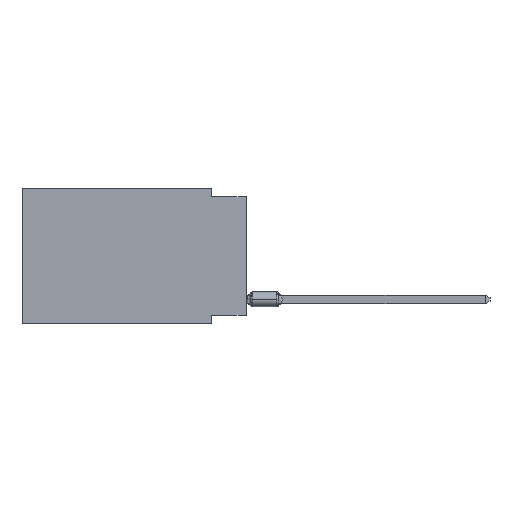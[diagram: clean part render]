
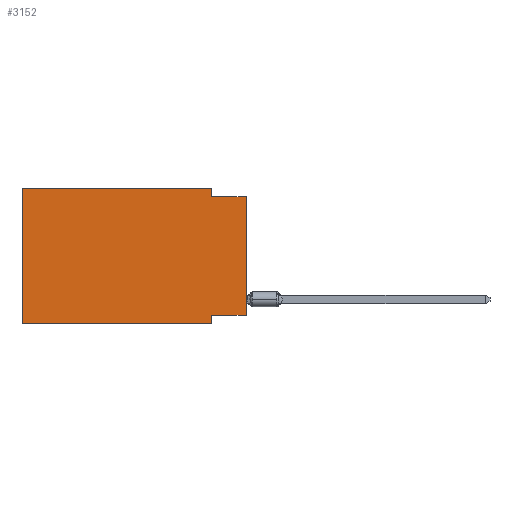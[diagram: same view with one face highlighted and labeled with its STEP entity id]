
A CAD part, left-side view. The second image highlights one B-rep face of the part: STEP entity #3152.
In plain terms, the highlighted planar face has unit normal (-1, 0, 0).
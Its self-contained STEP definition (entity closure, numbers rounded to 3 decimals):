
#295 = VERTEX_POINT ( 'NONE', #4815 ) ;
#475 = CARTESIAN_POINT ( 'NONE',  ( 0., 0., 0. ) ) ;
#758 = DIRECTION ( 'NONE',  ( 0., -1., 0. ) ) ;
#931 = VECTOR ( 'NONE', #13172, 1000. ) ;
#940 = CARTESIAN_POINT ( 'NONE',  ( 0., 16.383, 0. ) ) ;
#1069 = VECTOR ( 'NONE', #4047, 1000. ) ;
#1513 = LINE ( 'NONE', #475, #11340 ) ;
#2204 = VERTEX_POINT ( 'NONE', #8667 ) ;
#2489 = DIRECTION ( 'NONE',  ( 0., 0., -1. ) ) ;
#2542 = VECTOR ( 'NONE', #8967, 1000. ) ;
#3152 = ADVANCED_FACE ( 'NONE', ( #3897 ), #14091, .F. ) ;
#3255 = EDGE_CURVE ( 'NONE', #7846, #295, #1513, .T. ) ;
#3309 = CARTESIAN_POINT ( 'NONE',  ( 0., 0., -0.635 ) ) ;
#3440 = CARTESIAN_POINT ( 'NONE',  ( 0., 16.383, 0. ) ) ;
#3498 = CARTESIAN_POINT ( 'NONE',  ( 0., 16.383, 0. ) ) ;
#3897 = FACE_OUTER_BOUND ( 'NONE', #4303, .T. ) ;
#4021 = EDGE_CURVE ( 'NONE', #14570, #295, #4859, .T. ) ;
#4047 = DIRECTION ( 'NONE',  ( 0., 0., -1. ) ) ;
#4248 = VECTOR ( 'NONE', #12538, 1000. ) ;
#4303 = EDGE_LOOP ( 'NONE', ( #13614, #16220, #7814, #13101, #13898, #14642, #16338, #11580 ) ) ;
#4553 = DIRECTION ( 'NONE',  ( 0., 0., 1. ) ) ;
#4555 = VERTEX_POINT ( 'NONE', #12777 ) ;
#4815 = CARTESIAN_POINT ( 'NONE',  ( 0., 0., -0.635 ) ) ;
#4859 = LINE ( 'NONE', #3309, #4248 ) ;
#4900 = LINE ( 'NONE', #3440, #6877 ) ;
#6648 = DIRECTION ( 'NONE',  ( 0., 0., 1. ) ) ;
#6824 = EDGE_CURVE ( 'NONE', #14554, #16844, #4900, .T. ) ;
#6877 = VECTOR ( 'NONE', #4553, 1000. ) ;
#6938 = CARTESIAN_POINT ( 'NONE',  ( 0., 0., -9.271 ) ) ;
#7018 = LINE ( 'NONE', #9733, #13177 ) ;
#7523 = LINE ( 'NONE', #3498, #2542 ) ;
#7814 = ORIENTED_EDGE ( 'NONE', *, *, #16380, .F. ) ;
#7846 = VERTEX_POINT ( 'NONE', #11588 ) ;
#8667 = CARTESIAN_POINT ( 'NONE',  ( 0., 2.54, 0. ) ) ;
#8840 = VECTOR ( 'NONE', #2489, 1000. ) ;
#8967 = DIRECTION ( 'NONE',  ( 0., -1., 0. ) ) ;
#9119 = CARTESIAN_POINT ( 'NONE',  ( 0., 16.383, 0. ) ) ;
#9468 = EDGE_CURVE ( 'NONE', #14554, #4555, #7018, .T. ) ;
#9588 = EDGE_CURVE ( 'NONE', #16844, #2204, #7523, .T. ) ;
#9733 = CARTESIAN_POINT ( 'NONE',  ( 0., 16.383, -9.906 ) ) ;
#9786 = CARTESIAN_POINT ( 'NONE',  ( 0., 16.383, -9.906 ) ) ;
#9879 = VERTEX_POINT ( 'NONE', #10924 ) ;
#10101 = LINE ( 'NONE', #12832, #8840 ) ;
#10388 = CARTESIAN_POINT ( 'NONE',  ( 0., 2.54, -0.635 ) ) ;
#10816 = LINE ( 'NONE', #16103, #1069 ) ;
#10924 = CARTESIAN_POINT ( 'NONE',  ( 0., 2.54, -9.271 ) ) ;
#11340 = VECTOR ( 'NONE', #6648, 1000. ) ;
#11580 = ORIENTED_EDGE ( 'NONE', *, *, #16513, .F. ) ;
#11588 = CARTESIAN_POINT ( 'NONE',  ( 0., 0., -9.271 ) ) ;
#12060 = LINE ( 'NONE', #6938, #931 ) ;
#12302 = AXIS2_PLACEMENT_3D ( 'NONE', #9119, #14337, #12802 ) ;
#12538 = DIRECTION ( 'NONE',  ( 0., -1., 0. ) ) ;
#12777 = CARTESIAN_POINT ( 'NONE',  ( 0., 2.54, -9.906 ) ) ;
#12802 = DIRECTION ( 'NONE',  ( 0., 0., -1. ) ) ;
#12832 = CARTESIAN_POINT ( 'NONE',  ( 0., 2.54, 0. ) ) ;
#13101 = ORIENTED_EDGE ( 'NONE', *, *, #9588, .F. ) ;
#13172 = DIRECTION ( 'NONE',  ( 0., 1., 0. ) ) ;
#13177 = VECTOR ( 'NONE', #758, 1000. ) ;
#13449 = EDGE_CURVE ( 'NONE', #9879, #4555, #10816, .T. ) ;
#13614 = ORIENTED_EDGE ( 'NONE', *, *, #3255, .T. ) ;
#13898 = ORIENTED_EDGE ( 'NONE', *, *, #6824, .F. ) ;
#14091 = PLANE ( 'NONE',  #12302 ) ;
#14337 = DIRECTION ( 'NONE',  ( 1., 0., 0. ) ) ;
#14554 = VERTEX_POINT ( 'NONE', #9786 ) ;
#14570 = VERTEX_POINT ( 'NONE', #10388 ) ;
#14642 = ORIENTED_EDGE ( 'NONE', *, *, #9468, .T. ) ;
#16103 = CARTESIAN_POINT ( 'NONE',  ( 0., 2.54, -9.906 ) ) ;
#16220 = ORIENTED_EDGE ( 'NONE', *, *, #4021, .F. ) ;
#16338 = ORIENTED_EDGE ( 'NONE', *, *, #13449, .F. ) ;
#16380 = EDGE_CURVE ( 'NONE', #2204, #14570, #10101, .T. ) ;
#16513 = EDGE_CURVE ( 'NONE', #7846, #9879, #12060, .T. ) ;
#16844 = VERTEX_POINT ( 'NONE', #940 ) ;
